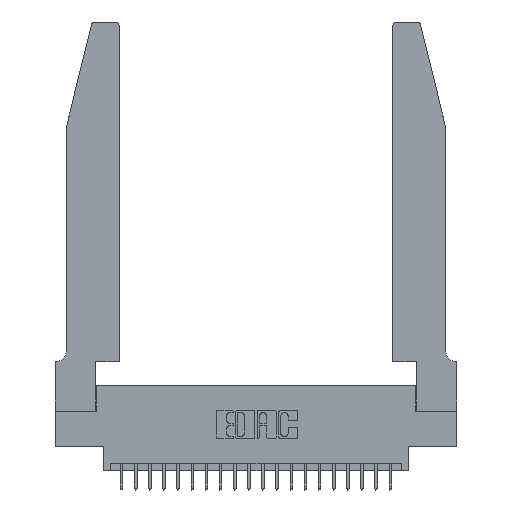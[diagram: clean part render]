
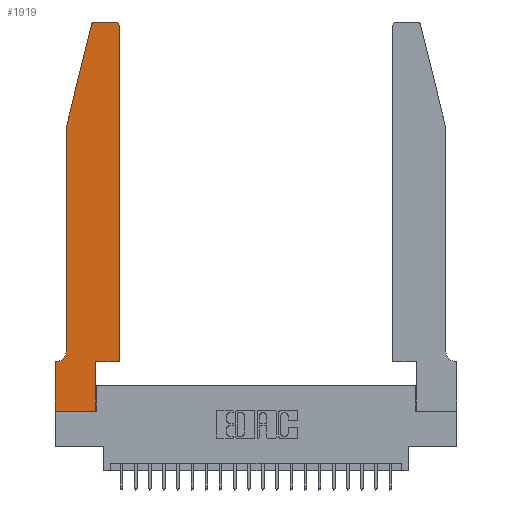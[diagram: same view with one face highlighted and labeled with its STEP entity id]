
A CAD part, top view. The second image highlights one B-rep face of the part: STEP entity #1919.
In plain terms, the highlighted planar face has unit normal (0, 0, 1).
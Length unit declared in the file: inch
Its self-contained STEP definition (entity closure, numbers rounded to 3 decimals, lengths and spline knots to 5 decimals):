
#81 = CIRCLE ( 'NONE', #7741, 0.03 ) ;
#635 = ORIENTED_EDGE ( 'NONE', *, *, #13596, .T. ) ;
#744 = DIRECTION ( 'NONE',  ( -0.239, -0.971, 0. ) ) ;
#1287 = CARTESIAN_POINT ( 'NONE',  ( 0.4505, 0.35, 0.37 ) ) ;
#1672 = VECTOR ( 'NONE', #8593, 39.37008 ) ;
#1919 = ADVANCED_FACE ( 'NONE', ( #20207 ), #2484, .T. ) ;
#1936 = VERTEX_POINT ( 'NONE', #16963 ) ;
#2261 = CARTESIAN_POINT ( 'NONE',  ( 0.0755, 0.35, 0.37 ) ) ;
#2365 = VECTOR ( 'NONE', #744, 39.37008 ) ;
#2390 = DIRECTION ( 'NONE',  ( 0., -1., 0. ) ) ;
#2475 = CARTESIAN_POINT ( 'NONE',  ( 0., 0., 0.37 ) ) ;
#2484 = PLANE ( 'NONE',  #12198 ) ;
#2528 = CARTESIAN_POINT ( 'NONE',  ( 0.2865, 0., 0.37 ) ) ;
#2689 = CARTESIAN_POINT ( 'NONE',  ( 0.0755, 0.42, 0.37 ) ) ;
#2772 = CIRCLE ( 'NONE', #11213, 0.07 ) ;
#2934 = DIRECTION ( 'NONE',  ( 1., 0., 0. ) ) ;
#2976 = EDGE_CURVE ( 'NONE', #6572, #11146, #3703, .T. ) ;
#2991 = DIRECTION ( 'NONE',  ( 1., 0., 0. ) ) ;
#3229 = EDGE_LOOP ( 'NONE', ( #16593, #14525, #9938, #17429, #11144, #22876, #5144, #12961, #635, #11337, #11697, #9862 ) ) ;
#3510 = EDGE_CURVE ( 'NONE', #1936, #18519, #81, .T. ) ;
#3703 = LINE ( 'NONE', #4062, #9946 ) ;
#4062 = CARTESIAN_POINT ( 'NONE',  ( 0.4505, 0.35, 0.37 ) ) ;
#4314 = AXIS2_PLACEMENT_3D ( 'NONE', #19331, #15656, #2934 ) ;
#4508 = EDGE_CURVE ( 'NONE', #22737, #12089, #2772, .T. ) ;
#5023 = VERTEX_POINT ( 'NONE', #17065 ) ;
#5115 = EDGE_CURVE ( 'NONE', #14989, #9988, #23452, .T. ) ;
#5144 = ORIENTED_EDGE ( 'NONE', *, *, #8480, .T. ) ;
#5171 = EDGE_CURVE ( 'NONE', #18519, #14989, #23063, .T. ) ;
#6080 = VECTOR ( 'NONE', #13178, 39.37008 ) ;
#6547 = CARTESIAN_POINT ( 'NONE',  ( 0.0055, 0.35, 0.37 ) ) ;
#6572 = VERTEX_POINT ( 'NONE', #7579 ) ;
#6581 = DIRECTION ( 'NONE',  ( 0., -1., 0. ) ) ;
#6599 = VECTOR ( 'NONE', #7052, 39.37008 ) ;
#6662 = DIRECTION ( 'NONE',  ( -1., 0., 0. ) ) ;
#6838 = CARTESIAN_POINT ( 'NONE',  ( 0.4205, 2.72, 0.37 ) ) ;
#7008 = DIRECTION ( 'NONE',  ( -1., 0., 0. ) ) ;
#7052 = DIRECTION ( 'NONE',  ( 1., 0., 0. ) ) ;
#7288 = CARTESIAN_POINT ( 'NONE',  ( 0., 0., 0.37 ) ) ;
#7398 = LINE ( 'NONE', #7288, #6599 ) ;
#7413 = EDGE_CURVE ( 'NONE', #19381, #8113, #7398, .T. ) ;
#7502 = VECTOR ( 'NONE', #18467, 39.37008 ) ;
#7547 = LINE ( 'NONE', #2261, #6080 ) ;
#7579 = CARTESIAN_POINT ( 'NONE',  ( 0.2865, 0.35, 0.37 ) ) ;
#7741 = AXIS2_PLACEMENT_3D ( 'NONE', #6838, #17719, #2991 ) ;
#8113 = VERTEX_POINT ( 'NONE', #2528 ) ;
#8392 = CARTESIAN_POINT ( 'NONE',  ( 0.0755, 2., 0.37 ) ) ;
#8475 = LINE ( 'NONE', #1287, #1672 ) ;
#8480 = EDGE_CURVE ( 'NONE', #17130, #19381, #20713, .T. ) ;
#8593 = DIRECTION ( 'NONE',  ( 0., 1., 0. ) ) ;
#8986 = EDGE_CURVE ( 'NONE', #11146, #1936, #8475, .T. ) ;
#9295 = VECTOR ( 'NONE', #6581, 39.37008 ) ;
#9435 = DIRECTION ( 'NONE',  ( 1., 0., 0. ) ) ;
#9633 = CARTESIAN_POINT ( 'NONE',  ( 0.2865, 0.35, 0.37 ) ) ;
#9862 = ORIENTED_EDGE ( 'NONE', *, *, #3510, .T. ) ;
#9938 = ORIENTED_EDGE ( 'NONE', *, *, #21410, .T. ) ;
#9946 = VECTOR ( 'NONE', #16428, 39.37008 ) ;
#9988 = VERTEX_POINT ( 'NONE', #16170 ) ;
#10186 = LINE ( 'NONE', #8392, #14804 ) ;
#11144 = ORIENTED_EDGE ( 'NONE', *, *, #4508, .T. ) ;
#11146 = VERTEX_POINT ( 'NONE', #19385 ) ;
#11213 = AXIS2_PLACEMENT_3D ( 'NONE', #15995, #16343, #7008 ) ;
#11337 = ORIENTED_EDGE ( 'NONE', *, *, #2976, .T. ) ;
#11608 = CARTESIAN_POINT ( 'NONE',  ( 0., 0., 0.37 ) ) ;
#11697 = ORIENTED_EDGE ( 'NONE', *, *, #8986, .T. ) ;
#12089 = VERTEX_POINT ( 'NONE', #6547 ) ;
#12198 = AXIS2_PLACEMENT_3D ( 'NONE', #18510, #20561, #9435 ) ;
#12291 = CARTESIAN_POINT ( 'NONE',  ( 0.2605, 2.75, 0.37 ) ) ;
#12961 = ORIENTED_EDGE ( 'NONE', *, *, #7413, .T. ) ;
#12997 = LINE ( 'NONE', #9633, #7502 ) ;
#13178 = DIRECTION ( 'NONE',  ( -1., 0., 0. ) ) ;
#13596 = EDGE_CURVE ( 'NONE', #8113, #6572, #12997, .T. ) ;
#14525 = ORIENTED_EDGE ( 'NONE', *, *, #5115, .T. ) ;
#14804 = VECTOR ( 'NONE', #2390, 39.37008 ) ;
#14989 = VERTEX_POINT ( 'NONE', #14992 ) ;
#14992 = CARTESIAN_POINT ( 'NONE',  ( 0.284, 2.75, 0.37 ) ) ;
#15138 = EDGE_CURVE ( 'NONE', #5023, #22737, #10186, .T. ) ;
#15656 = DIRECTION ( 'NONE',  ( 0., 0., 1. ) ) ;
#15995 = CARTESIAN_POINT ( 'NONE',  ( 0.0055, 0.42, 0.37 ) ) ;
#16170 = CARTESIAN_POINT ( 'NONE',  ( 0.25487, 2.72718, 0.37 ) ) ;
#16343 = DIRECTION ( 'NONE',  ( 0., 0., -1. ) ) ;
#16428 = DIRECTION ( 'NONE',  ( 1., 0., 0. ) ) ;
#16593 = ORIENTED_EDGE ( 'NONE', *, *, #5171, .T. ) ;
#16963 = CARTESIAN_POINT ( 'NONE',  ( 0.4505, 2.72, 0.37 ) ) ;
#17065 = CARTESIAN_POINT ( 'NONE',  ( 0.0755, 2., 0.37 ) ) ;
#17130 = VERTEX_POINT ( 'NONE', #18963 ) ;
#17429 = ORIENTED_EDGE ( 'NONE', *, *, #15138, .T. ) ;
#17719 = DIRECTION ( 'NONE',  ( 0., 0., 1. ) ) ;
#18467 = DIRECTION ( 'NONE',  ( 0., 1., 0. ) ) ;
#18510 = CARTESIAN_POINT ( 'NONE',  ( 0., 0.35, 0.37 ) ) ;
#18519 = VERTEX_POINT ( 'NONE', #19030 ) ;
#18828 = EDGE_CURVE ( 'NONE', #12089, #17130, #7547, .T. ) ;
#18963 = CARTESIAN_POINT ( 'NONE',  ( 0., 0.35, 0.37 ) ) ;
#19030 = CARTESIAN_POINT ( 'NONE',  ( 0.4205, 2.75, 0.37 ) ) ;
#19163 = LINE ( 'NONE', #20982, #2365 ) ;
#19331 = CARTESIAN_POINT ( 'NONE',  ( 0.284, 2.72, 0.37 ) ) ;
#19381 = VERTEX_POINT ( 'NONE', #2475 ) ;
#19385 = CARTESIAN_POINT ( 'NONE',  ( 0.4505, 0.35, 0.37 ) ) ;
#20007 = VECTOR ( 'NONE', #6662, 39.37008 ) ;
#20207 = FACE_OUTER_BOUND ( 'NONE', #3229, .T. ) ;
#20561 = DIRECTION ( 'NONE',  ( 0., 0., 1. ) ) ;
#20713 = LINE ( 'NONE', #11608, #9295 ) ;
#20982 = CARTESIAN_POINT ( 'NONE',  ( 0.0755, 2., 0.37 ) ) ;
#21410 = EDGE_CURVE ( 'NONE', #9988, #5023, #19163, .T. ) ;
#22737 = VERTEX_POINT ( 'NONE', #2689 ) ;
#22876 = ORIENTED_EDGE ( 'NONE', *, *, #18828, .T. ) ;
#23063 = LINE ( 'NONE', #12291, #20007 ) ;
#23452 = CIRCLE ( 'NONE', #4314, 0.03 ) ;
